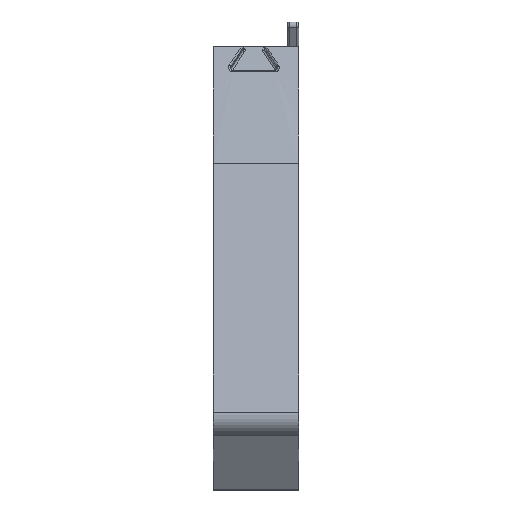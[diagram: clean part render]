
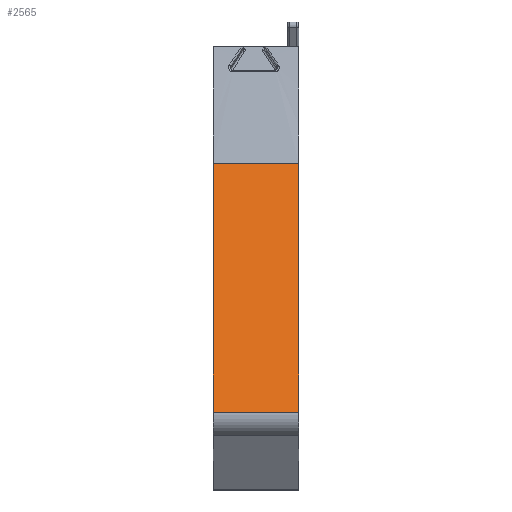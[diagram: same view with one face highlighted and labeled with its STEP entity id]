
A CAD part, left-side view. The second image highlights one B-rep face of the part: STEP entity #2565.
In plain terms, the highlighted planar face has unit normal (-0.961, 0, 0.276).
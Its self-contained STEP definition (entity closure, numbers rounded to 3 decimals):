
#365=FACE_OUTER_BOUND('',#516,.T.);
#516=EDGE_LOOP('',(#2168,#2169,#2170,#2171));
#670=LINE('',#3946,#855);
#741=LINE('',#5123,#926);
#746=LINE('',#5203,#931);
#747=LINE('',#5204,#932);
#855=VECTOR('',#3011,10.);
#926=VECTOR('',#3386,10.);
#931=VECTOR('',#3425,10.);
#932=VECTOR('',#3426,10.);
#1076=VERTEX_POINT('',#3943);
#1077=VERTEX_POINT('',#3945);
#1165=VERTEX_POINT('',#5121);
#1175=VERTEX_POINT('',#5202);
#1322=EDGE_CURVE('',#1076,#1077,#670,.T.);
#1504=EDGE_CURVE('',#1076,#1165,#741,.T.);
#1522=EDGE_CURVE('',#1165,#1175,#746,.T.);
#1523=EDGE_CURVE('',#1077,#1175,#747,.T.);
#2168=ORIENTED_EDGE('',*,*,#1504,.T.);
#2169=ORIENTED_EDGE('',*,*,#1522,.T.);
#2170=ORIENTED_EDGE('',*,*,#1523,.F.);
#2171=ORIENTED_EDGE('',*,*,#1322,.F.);
#2437=PLANE('',#2822);
#2565=ADVANCED_FACE('',(#365),#2437,.T.);
#2822=AXIS2_PLACEMENT_3D('',#5201,#3423,#3424);
#3011=DIRECTION('',(-0.276,0.,-0.961));
#3386=DIRECTION('',(0.,1.,0.));
#3423=DIRECTION('center_axis',(-0.961,0.,
0.276));
#3424=DIRECTION('ref_axis',(0.,1.,0.));
#3425=DIRECTION('',(-0.276,0.,-0.961));
#3426=DIRECTION('',(0.,1.,0.));
#3943=CARTESIAN_POINT('',(-145.174,6.11,-285.844));
#3945=CARTESIAN_POINT('',(-173.147,6.11,-383.398));
#3946=CARTESIAN_POINT('',(-145.912,6.11,-288.418));
#5121=CARTESIAN_POINT('',(-145.174,39.734,-285.844));
#5123=CARTESIAN_POINT('',(-145.174,39.734,-285.844));
#5201=CARTESIAN_POINT('Origin',(-145.174,6.118,-285.844));
#5202=CARTESIAN_POINT('',(-173.147,39.734,-383.398));
#5203=CARTESIAN_POINT('',(-145.174,39.734,-285.844));
#5204=CARTESIAN_POINT('',(-173.147,14.522,-383.398));
